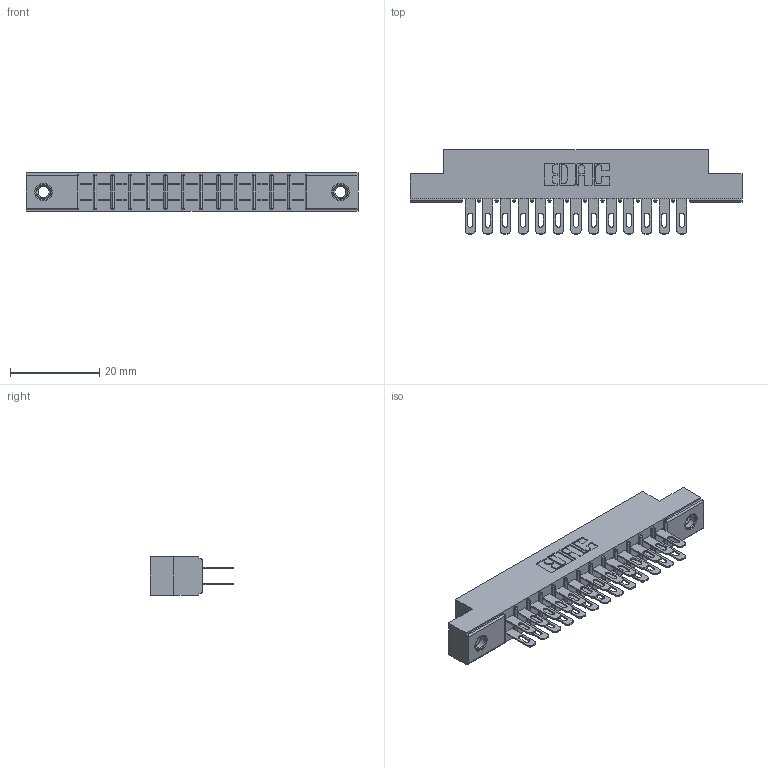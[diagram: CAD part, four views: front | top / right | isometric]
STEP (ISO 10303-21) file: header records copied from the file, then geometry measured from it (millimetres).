
FILE_DESCRIPTION (( 'STEP AP203' ), '1' );
FILE_NAME ('305-026-500-507.STEP', '2019-09-09T15:05:20', ( '' ), ( '' ), 'SwSTEP 2.0', 'SolidWorks 2016', '' );
FILE_SCHEMA (( 'CONFIG_CONTROL_DESIGN' ));
Length unit declared in the file: inch
Products named in the file (4): 305-290-001_500; 305 Part_.156 Dia; 305-026-500-507; 345-250-001_345-250-005-103
Assembly tree (29 placements, depth 2):
  305-026-500-507
    305 Part_.156 Dia
    305-290-001_500  x26
    345-250-001_345-250-005-103  x2
Bounding box: 74.52 x 18.85 x 8.71 mm (x, y, z)
Volume: 4568.1 mm3; surface area: 9015.2 mm2
Topology: 29 solids, 29 shells, 1476 faces, 4183 edges, 2710 vertices
Faces by surface type: plane 828, cylinder 580, sphere 52, cone 12, torus 4
Entity records: 18813 total; most frequent: CARTESIAN_POINT 3096, ORIENTED_EDGE 3062, DIRECTION 3031, EDGE_CURVE 1531, VECTOR 1201, LINE 1201, VERTEX_POINT 980, AXIS2_PLACEMENT_3D 915
